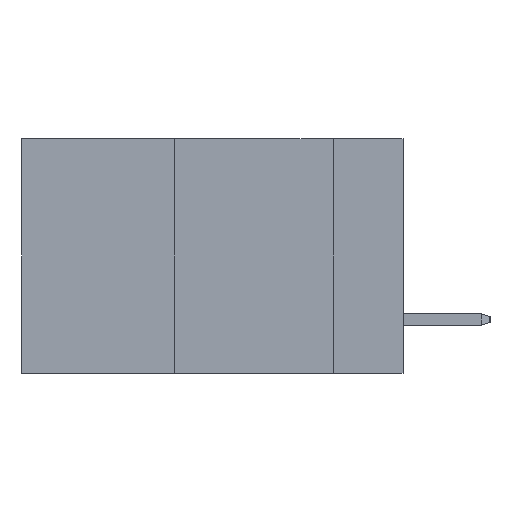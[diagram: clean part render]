
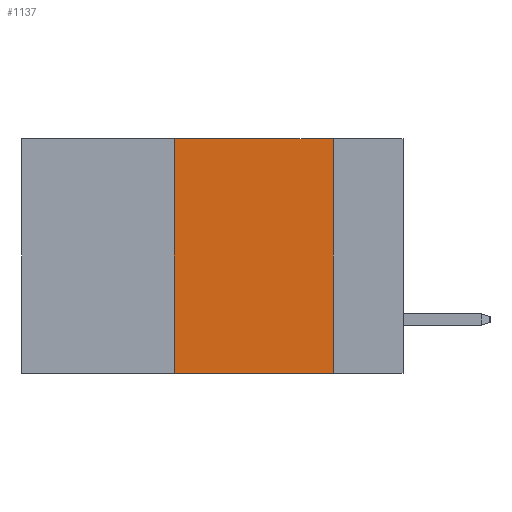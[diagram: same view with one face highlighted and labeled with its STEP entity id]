
A CAD part, left-side view. The second image highlights one B-rep face of the part: STEP entity #1137.
In plain terms, the highlighted planar face has unit normal (-1, 0, 0).
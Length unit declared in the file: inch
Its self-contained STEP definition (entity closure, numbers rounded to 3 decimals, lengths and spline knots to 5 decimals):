
#34 = EDGE_LOOP ( 'NONE', ( #11571, #1857, #5305, #8750 ) ) ;
#581 = VECTOR ( 'NONE', #2309, 39.37008 ) ;
#1137 = ADVANCED_FACE ( 'NONE', ( #20762 ), #16480, .F. ) ;
#1857 = ORIENTED_EDGE ( 'NONE', *, *, #17849, .F. ) ;
#2309 = DIRECTION ( 'NONE',  ( 0., -1., 0. ) ) ;
#2985 = CARTESIAN_POINT ( 'NONE',  ( 0., 0.6, 0. ) ) ;
#3728 = CARTESIAN_POINT ( 'NONE',  ( 0., 0.11, 0. ) ) ;
#4811 = VERTEX_POINT ( 'NONE', #13610 ) ;
#5074 = VECTOR ( 'NONE', #18576, 39.37008 ) ;
#5160 = CARTESIAN_POINT ( 'NONE',  ( 0., 0.36, 0. ) ) ;
#5305 = ORIENTED_EDGE ( 'NONE', *, *, #11000, .F. ) ;
#5773 = LINE ( 'NONE', #13691, #21010 ) ;
#5885 = LINE ( 'NONE', #17827, #11627 ) ;
#6372 = DIRECTION ( 'NONE',  ( 0., 0., -1. ) ) ;
#7678 = VERTEX_POINT ( 'NONE', #5160 ) ;
#8718 = CARTESIAN_POINT ( 'NONE',  ( 0., 0.36, 0. ) ) ;
#8750 = ORIENTED_EDGE ( 'NONE', *, *, #21526, .T. ) ;
#9203 = EDGE_CURVE ( 'NONE', #24403, #4811, #5885, .T. ) ;
#9959 = VERTEX_POINT ( 'NONE', #17482 ) ;
#11000 = EDGE_CURVE ( 'NONE', #9959, #7678, #22327, .T. ) ;
#11571 = ORIENTED_EDGE ( 'NONE', *, *, #9203, .F. ) ;
#11627 = VECTOR ( 'NONE', #23788, 39.37008 ) ;
#11928 = LINE ( 'NONE', #14249, #581 ) ;
#12120 = DIRECTION ( 'NONE',  ( 0., -1., 0. ) ) ;
#12734 = DIRECTION ( 'NONE',  ( 1., 0., 0. ) ) ;
#13610 = CARTESIAN_POINT ( 'NONE',  ( 0., 0.11, -0.37 ) ) ;
#13691 = CARTESIAN_POINT ( 'NONE',  ( 0., 0.6, 0. ) ) ;
#14249 = CARTESIAN_POINT ( 'NONE',  ( 0., 0.6, -0.37 ) ) ;
#16480 = PLANE ( 'NONE',  #21314 ) ;
#17482 = CARTESIAN_POINT ( 'NONE',  ( 0., 0.36, -0.37 ) ) ;
#17827 = CARTESIAN_POINT ( 'NONE',  ( 0., 0.11, 0. ) ) ;
#17849 = EDGE_CURVE ( 'NONE', #7678, #24403, #5773, .T. ) ;
#18576 = DIRECTION ( 'NONE',  ( 0., 0., 1. ) ) ;
#20762 = FACE_OUTER_BOUND ( 'NONE', #34, .T. ) ;
#21010 = VECTOR ( 'NONE', #12120, 39.37008 ) ;
#21314 = AXIS2_PLACEMENT_3D ( 'NONE', #2985, #12734, #6372 ) ;
#21526 = EDGE_CURVE ( 'NONE', #9959, #4811, #11928, .T. ) ;
#22327 = LINE ( 'NONE', #8718, #5074 ) ;
#23788 = DIRECTION ( 'NONE',  ( 0., 0., -1. ) ) ;
#24403 = VERTEX_POINT ( 'NONE', #3728 ) ;
